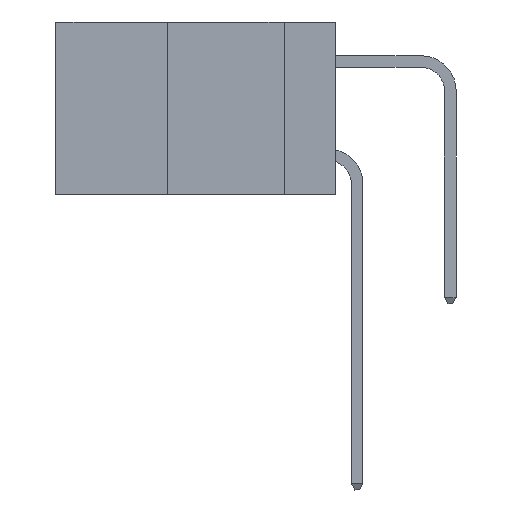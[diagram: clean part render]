
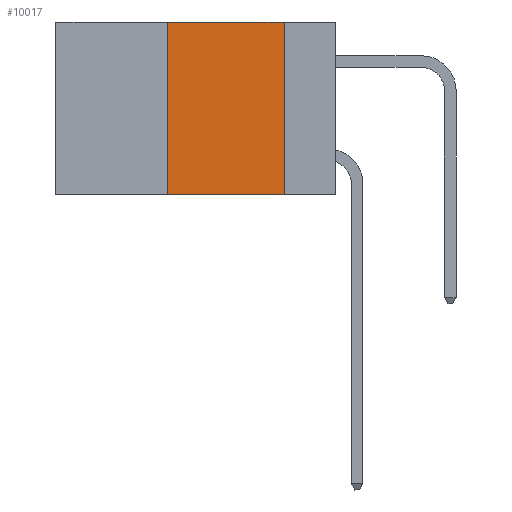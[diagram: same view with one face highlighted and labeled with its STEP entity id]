
A CAD part, left-side view. The second image highlights one B-rep face of the part: STEP entity #10017.
In plain terms, the highlighted planar face has unit normal (-1, 0, 0).
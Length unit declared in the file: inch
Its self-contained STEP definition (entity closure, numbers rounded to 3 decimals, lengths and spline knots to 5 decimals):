
#1074 = CARTESIAN_POINT ( 'NONE',  ( 0., 0.11, 0. ) ) ;
#2369 = CARTESIAN_POINT ( 'NONE',  ( 0., 0.6, -0.37 ) ) ;
#4520 = VECTOR ( 'NONE', #22239, 39.37008 ) ;
#5010 = ORIENTED_EDGE ( 'NONE', *, *, #20153, .T. ) ;
#5231 = LINE ( 'NONE', #1074, #4520 ) ;
#5296 = EDGE_LOOP ( 'NONE', ( #16841, #22813, #13360, #5010 ) ) ;
#5677 = AXIS2_PLACEMENT_3D ( 'NONE', #27108, #29290, #10925 ) ;
#5871 = LINE ( 'NONE', #28180, #24821 ) ;
#6415 = CARTESIAN_POINT ( 'NONE',  ( 0., 0.36, -0.37 ) ) ;
#7509 = DIRECTION ( 'NONE',  ( 0., -1., 0. ) ) ;
#9790 = VERTEX_POINT ( 'NONE', #9958 ) ;
#9958 = CARTESIAN_POINT ( 'NONE',  ( 0., 0.11, 0. ) ) ;
#10017 = ADVANCED_FACE ( 'NONE', ( #26704 ), #20244, .F. ) ;
#10384 = EDGE_CURVE ( 'NONE', #9790, #21735, #5231, .T. ) ;
#10925 = DIRECTION ( 'NONE',  ( 0., 0., -1. ) ) ;
#11070 = VECTOR ( 'NONE', #18567, 39.37008 ) ;
#11759 = VECTOR ( 'NONE', #16204, 39.37008 ) ;
#12649 = CARTESIAN_POINT ( 'NONE',  ( 0., 0.36, 0. ) ) ;
#13360 = ORIENTED_EDGE ( 'NONE', *, *, #13723, .F. ) ;
#13723 = EDGE_CURVE ( 'NONE', #14891, #29375, #22540, .T. ) ;
#13916 = CARTESIAN_POINT ( 'NONE',  ( 0., 0.36, 0. ) ) ;
#14891 = VERTEX_POINT ( 'NONE', #6415 ) ;
#15747 = LINE ( 'NONE', #2369, #11759 ) ;
#16204 = DIRECTION ( 'NONE',  ( 0., -1., 0. ) ) ;
#16841 = ORIENTED_EDGE ( 'NONE', *, *, #10384, .F. ) ;
#17214 = EDGE_CURVE ( 'NONE', #29375, #9790, #5871, .T. ) ;
#18567 = DIRECTION ( 'NONE',  ( 0., 0., 1. ) ) ;
#20153 = EDGE_CURVE ( 'NONE', #14891, #21735, #15747, .T. ) ;
#20244 = PLANE ( 'NONE',  #5677 ) ;
#20675 = CARTESIAN_POINT ( 'NONE',  ( 0., 0.11, -0.37 ) ) ;
#21735 = VERTEX_POINT ( 'NONE', #20675 ) ;
#22239 = DIRECTION ( 'NONE',  ( 0., 0., -1. ) ) ;
#22540 = LINE ( 'NONE', #13916, #11070 ) ;
#22813 = ORIENTED_EDGE ( 'NONE', *, *, #17214, .F. ) ;
#24821 = VECTOR ( 'NONE', #7509, 39.37008 ) ;
#26704 = FACE_OUTER_BOUND ( 'NONE', #5296, .T. ) ;
#27108 = CARTESIAN_POINT ( 'NONE',  ( 0., 0.6, 0. ) ) ;
#28180 = CARTESIAN_POINT ( 'NONE',  ( 0., 0.6, 0. ) ) ;
#29290 = DIRECTION ( 'NONE',  ( 1., 0., 0. ) ) ;
#29375 = VERTEX_POINT ( 'NONE', #12649 ) ;
